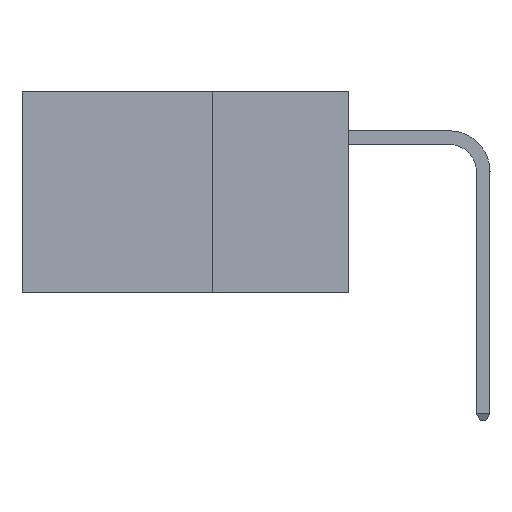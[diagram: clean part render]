
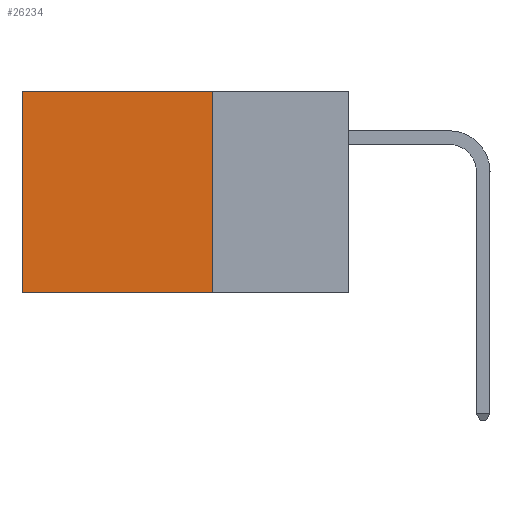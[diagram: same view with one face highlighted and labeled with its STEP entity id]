
A CAD part, left-side view. The second image highlights one B-rep face of the part: STEP entity #26234.
In plain terms, the highlighted planar face has unit normal (-1, 0, 0).
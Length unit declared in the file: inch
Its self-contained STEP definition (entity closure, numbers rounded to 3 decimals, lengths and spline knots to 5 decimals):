
#314 = CARTESIAN_POINT ( 'NONE',  ( 0.2875, 0.6, -0.37 ) ) ;
#1213 = VERTEX_POINT ( 'NONE', #24994 ) ;
#4288 = PLANE ( 'NONE',  #22717 ) ;
#5243 = DIRECTION ( 'NONE',  ( 0., 0., -1. ) ) ;
#5732 = VECTOR ( 'NONE', #5243, 39.37008 ) ;
#8090 = DIRECTION ( 'NONE',  ( 1., 0., 0. ) ) ;
#10772 = EDGE_CURVE ( 'NONE', #1213, #26215, #23526, .T. ) ;
#15334 = CARTESIAN_POINT ( 'NONE',  ( 0.2875, 0.6, 0. ) ) ;
#17739 = LINE ( 'NONE', #35830, #36651 ) ;
#19789 = EDGE_CURVE ( 'NONE', #41236, #1213, #23857, .T. ) ;
#22502 = CARTESIAN_POINT ( 'NONE',  ( 0.2875, 0.25, 0. ) ) ;
#22717 = AXIS2_PLACEMENT_3D ( 'NONE', #34422, #8090, #34584 ) ;
#23526 = LINE ( 'NONE', #15334, #42374 ) ;
#23665 = ORIENTED_EDGE ( 'NONE', *, *, #48577, .F. ) ;
#23857 = LINE ( 'NONE', #22502, #42715 ) ;
#24994 = CARTESIAN_POINT ( 'NONE',  ( 0.2875, 0.6, 0. ) ) ;
#25644 = VERTEX_POINT ( 'NONE', #30707 ) ;
#26215 = VERTEX_POINT ( 'NONE', #314 ) ;
#26234 = ADVANCED_FACE ( 'NONE', ( #38227 ), #4288, .F. ) ;
#30707 = CARTESIAN_POINT ( 'NONE',  ( 0.2875, 0.25, -0.37 ) ) ;
#33081 = ORIENTED_EDGE ( 'NONE', *, *, #46916, .F. ) ;
#34422 = CARTESIAN_POINT ( 'NONE',  ( 0.2875, 0.25, 0. ) ) ;
#34584 = DIRECTION ( 'NONE',  ( 0., 0., -1. ) ) ;
#35830 = CARTESIAN_POINT ( 'NONE',  ( 0.2875, 0.25, -0.37 ) ) ;
#35942 = LINE ( 'NONE', #42102, #5732 ) ;
#36651 = VECTOR ( 'NONE', #39611, 39.37008 ) ;
#37668 = DIRECTION ( 'NONE',  ( 0., 1., 0. ) ) ;
#38227 = FACE_OUTER_BOUND ( 'NONE', #47468, .T. ) ;
#39611 = DIRECTION ( 'NONE',  ( 0., 1., 0. ) ) ;
#41236 = VERTEX_POINT ( 'NONE', #47839 ) ;
#41817 = DIRECTION ( 'NONE',  ( 0., 0., -1. ) ) ;
#42102 = CARTESIAN_POINT ( 'NONE',  ( 0.2875, 0.25, 0. ) ) ;
#42374 = VECTOR ( 'NONE', #41817, 39.37008 ) ;
#42715 = VECTOR ( 'NONE', #37668, 39.37008 ) ;
#45884 = ORIENTED_EDGE ( 'NONE', *, *, #10772, .T. ) ;
#46538 = ORIENTED_EDGE ( 'NONE', *, *, #19789, .T. ) ;
#46916 = EDGE_CURVE ( 'NONE', #25644, #26215, #17739, .T. ) ;
#47468 = EDGE_LOOP ( 'NONE', ( #45884, #33081, #23665, #46538 ) ) ;
#47839 = CARTESIAN_POINT ( 'NONE',  ( 0.2875, 0.25, 0. ) ) ;
#48577 = EDGE_CURVE ( 'NONE', #41236, #25644, #35942, .T. ) ;
